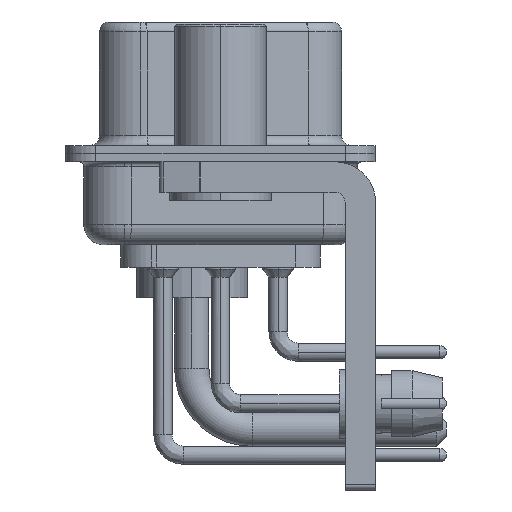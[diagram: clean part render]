
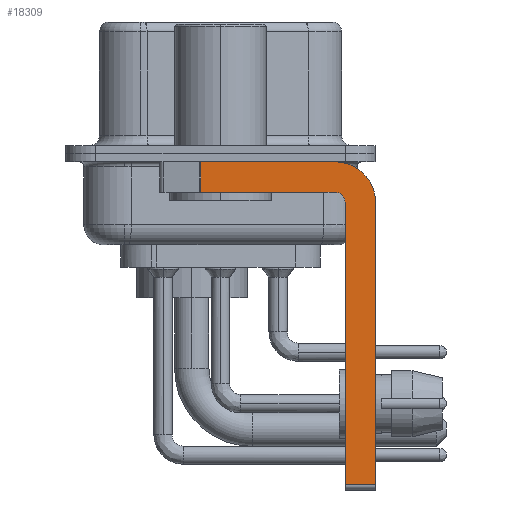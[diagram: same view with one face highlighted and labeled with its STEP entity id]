
A CAD part, left-side view. The second image highlights one B-rep face of the part: STEP entity #18309.
In plain terms, the highlighted planar face has unit normal (-1, 0, 0).
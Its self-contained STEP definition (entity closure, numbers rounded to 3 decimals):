
#77 = CARTESIAN_POINT ( 'NONE',  ( -2.9, -6.15, -16.35 ) ) ;
#571 = DIRECTION ( 'NONE',  ( 0., 0., -1. ) ) ;
#981 = VERTEX_POINT ( 'NONE', #21184 ) ;
#1134 = ORIENTED_EDGE ( 'NONE', *, *, #36742, .T. ) ;
#1269 = ORIENTED_EDGE ( 'NONE', *, *, #24153, .F. ) ;
#3292 = AXIS2_PLACEMENT_3D ( 'NONE', #18905, #21983, #22180 ) ;
#3634 = LINE ( 'NONE', #29162, #19577 ) ;
#3838 = VECTOR ( 'NONE', #16007, 1000. ) ;
#3972 = CARTESIAN_POINT ( 'NONE',  ( -2.9, -7.65, -16.35 ) ) ;
#4471 = DIRECTION ( 'NONE',  ( 0., 0., 1. ) ) ;
#4554 = ORIENTED_EDGE ( 'NONE', *, *, #30143, .F. ) ;
#4825 = ORIENTED_EDGE ( 'NONE', *, *, #30033, .F. ) ;
#5672 = VERTEX_POINT ( 'NONE', #36586 ) ;
#6164 = LINE ( 'NONE', #31293, #35587 ) ;
#6406 = LINE ( 'NONE', #21934, #3838 ) ;
#8150 = DIRECTION ( 'NONE',  ( -1., 0., 0. ) ) ;
#8708 = CARTESIAN_POINT ( 'NONE',  ( -2.9, 0.978, -1.9 ) ) ;
#9069 = EDGE_CURVE ( 'NONE', #24120, #13223, #6164, .T. ) ;
#9470 = AXIS2_PLACEMENT_3D ( 'NONE', #24046, #17319, #23454 ) ;
#10161 = VERTEX_POINT ( 'NONE', #3972 ) ;
#13223 = VERTEX_POINT ( 'NONE', #8708 ) ;
#13257 = LINE ( 'NONE', #31646, #14790 ) ;
#14790 = VECTOR ( 'NONE', #34307, 1000. ) ;
#15214 = DIRECTION ( 'NONE',  ( 0., -1., 0. ) ) ;
#16007 = DIRECTION ( 'NONE',  ( 0., 0., -1. ) ) ;
#16249 = CARTESIAN_POINT ( 'NONE',  ( -2.9, -6.15, -2.4 ) ) ;
#16290 = EDGE_CURVE ( 'NONE', #18783, #10161, #21731, .T. ) ;
#16395 = ORIENTED_EDGE ( 'NONE', *, *, #9069, .F. ) ;
#17237 = ORIENTED_EDGE ( 'NONE', *, *, #16290, .T. ) ;
#17319 = DIRECTION ( 'NONE',  ( 1., 0., 0. ) ) ;
#17764 = CARTESIAN_POINT ( 'NONE',  ( -2.9, 3., -0.4 ) ) ;
#18309 = ADVANCED_FACE ( 'NONE', ( #33826 ), #26902, .F. ) ;
#18783 = VERTEX_POINT ( 'NONE', #77 ) ;
#18905 = CARTESIAN_POINT ( 'NONE',  ( -2.9, -5.65, -2.4 ) ) ;
#19190 = EDGE_LOOP ( 'NONE', ( #4825, #1134, #16395, #32863, #4554, #17237, #34339, #1269 ) ) ;
#19577 = VECTOR ( 'NONE', #571, 1000. ) ;
#20199 = CARTESIAN_POINT ( 'NONE',  ( -2.9, -5.65, -2.4 ) ) ;
#21184 = CARTESIAN_POINT ( 'NONE',  ( -2.9, -7.65, -2.4 ) ) ;
#21305 = CIRCLE ( 'NONE', #34979, 0.5 ) ;
#21731 = LINE ( 'NONE', #30724, #26746 ) ;
#21934 = CARTESIAN_POINT ( 'NONE',  ( -2.9, -7.65, -2.4 ) ) ;
#21983 = DIRECTION ( 'NONE',  ( 1., 0., 0. ) ) ;
#22100 = DIRECTION ( 'NONE',  ( 0., 1., 0. ) ) ;
#22180 = DIRECTION ( 'NONE',  ( 0., 0., -1. ) ) ;
#23454 = DIRECTION ( 'NONE',  ( 0., 0., -1. ) ) ;
#24046 = CARTESIAN_POINT ( 'NONE',  ( -2.9, -5.65, -2.4 ) ) ;
#24120 = VERTEX_POINT ( 'NONE', #38778 ) ;
#24153 = EDGE_CURVE ( 'NONE', #28450, #981, #26425, .T. ) ;
#25347 = CARTESIAN_POINT ( 'NONE',  ( -2.9, -5.65, -0.4 ) ) ;
#26425 = CIRCLE ( 'NONE', #9470, 2. ) ;
#26746 = VECTOR ( 'NONE', #15214, 1000. ) ;
#26902 = PLANE ( 'NONE',  #3292 ) ;
#28450 = VERTEX_POINT ( 'NONE', #25347 ) ;
#29162 = CARTESIAN_POINT ( 'NONE',  ( -2.9, 0.978, -1.9 ) ) ;
#30033 = EDGE_CURVE ( 'NONE', #5672, #28450, #40253, .T. ) ;
#30143 = EDGE_CURVE ( 'NONE', #18783, #38499, #13257, .T. ) ;
#30240 = DIRECTION ( 'NONE',  ( 0., -1., 0. ) ) ;
#30724 = CARTESIAN_POINT ( 'NONE',  ( -2.9, -5.65, -16.35 ) ) ;
#31293 = CARTESIAN_POINT ( 'NONE',  ( -2.9, -5.65, -1.9 ) ) ;
#31646 = CARTESIAN_POINT ( 'NONE',  ( -2.9, -6.15, -16.6 ) ) ;
#31808 = EDGE_CURVE ( 'NONE', #38499, #24120, #21305, .T. ) ;
#32863 = ORIENTED_EDGE ( 'NONE', *, *, #31808, .F. ) ;
#33826 = FACE_OUTER_BOUND ( 'NONE', #19190, .T. ) ;
#33863 = EDGE_CURVE ( 'NONE', #981, #10161, #6406, .T. ) ;
#34307 = DIRECTION ( 'NONE',  ( 0., 0., 1. ) ) ;
#34339 = ORIENTED_EDGE ( 'NONE', *, *, #33863, .F. ) ;
#34979 = AXIS2_PLACEMENT_3D ( 'NONE', #20199, #8150, #4471 ) ;
#35587 = VECTOR ( 'NONE', #22100, 1000. ) ;
#36586 = CARTESIAN_POINT ( 'NONE',  ( -2.9, 0.978, -0.4 ) ) ;
#36742 = EDGE_CURVE ( 'NONE', #5672, #13223, #3634, .T. ) ;
#37575 = VECTOR ( 'NONE', #30240, 1000. ) ;
#38499 = VERTEX_POINT ( 'NONE', #16249 ) ;
#38778 = CARTESIAN_POINT ( 'NONE',  ( -2.9, -5.65, -1.9 ) ) ;
#40253 = LINE ( 'NONE', #17764, #37575 ) ;
